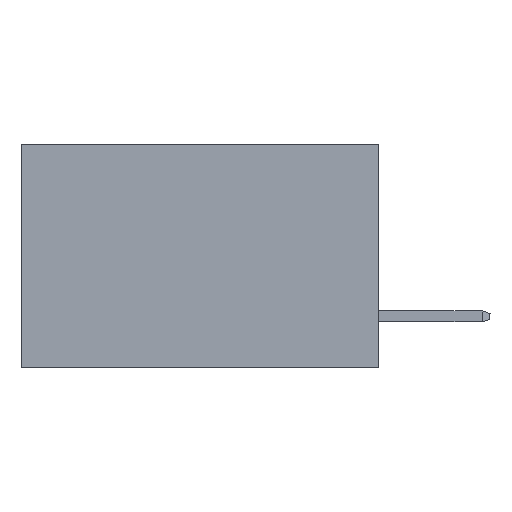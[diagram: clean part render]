
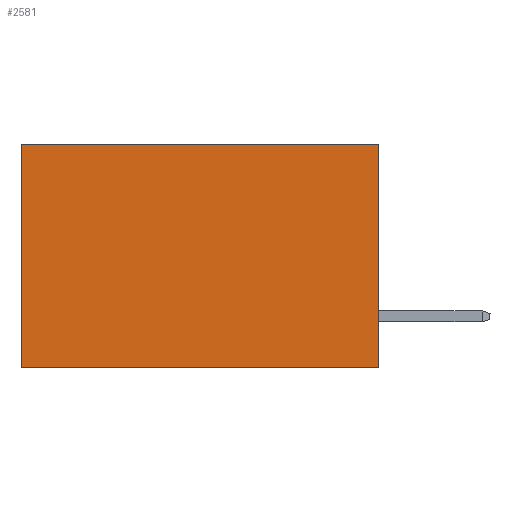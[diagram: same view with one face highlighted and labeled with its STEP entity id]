
A CAD part, left-side view. The second image highlights one B-rep face of the part: STEP entity #2581.
In plain terms, the highlighted planar face has unit normal (-1, 0, 0).
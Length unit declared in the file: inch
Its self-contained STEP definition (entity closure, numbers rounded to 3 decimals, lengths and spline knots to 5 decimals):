
#234 = VECTOR ( 'NONE', #2726, 39.37008 ) ;
#362 = LINE ( 'NONE', #3581, #11750 ) ;
#1575 = CARTESIAN_POINT ( 'NONE',  ( 0.277, 0.59, -0.37 ) ) ;
#2105 = CARTESIAN_POINT ( 'NONE',  ( 0.277, 0., -0.37 ) ) ;
#2530 = LINE ( 'NONE', #1575, #12619 ) ;
#2581 = ADVANCED_FACE ( 'NONE', ( #6671 ), #10044, .F. ) ;
#2726 = DIRECTION ( 'NONE',  ( 0., 1., 0. ) ) ;
#2768 = CARTESIAN_POINT ( 'NONE',  ( 0.277, 0., -0.37 ) ) ;
#3108 = DIRECTION ( 'NONE',  ( 1., 0., 0. ) ) ;
#3581 = CARTESIAN_POINT ( 'NONE',  ( 0.277, 0., 0. ) ) ;
#3671 = ORIENTED_EDGE ( 'NONE', *, *, #13797, .T. ) ;
#4850 = VERTEX_POINT ( 'NONE', #13586 ) ;
#5999 = DIRECTION ( 'NONE',  ( 0., 0., -1. ) ) ;
#6671 = FACE_OUTER_BOUND ( 'NONE', #15128, .T. ) ;
#9146 = ORIENTED_EDGE ( 'NONE', *, *, #15435, .T. ) ;
#9455 = VECTOR ( 'NONE', #5999, 39.37008 ) ;
#9879 = EDGE_CURVE ( 'NONE', #17568, #17441, #11213, .T. ) ;
#10044 = PLANE ( 'NONE',  #16343 ) ;
#11213 = LINE ( 'NONE', #2768, #234 ) ;
#11366 = CARTESIAN_POINT ( 'NONE',  ( 0.277, 0., 0. ) ) ;
#11750 = VECTOR ( 'NONE', #13020, 39.37008 ) ;
#12528 = DIRECTION ( 'NONE',  ( 0., 0., -1. ) ) ;
#12619 = VECTOR ( 'NONE', #12528, 39.37008 ) ;
#13012 = LINE ( 'NONE', #15502, #9455 ) ;
#13020 = DIRECTION ( 'NONE',  ( 0., 1., 0. ) ) ;
#13586 = CARTESIAN_POINT ( 'NONE',  ( 0.277, 0.59, 0. ) ) ;
#13797 = EDGE_CURVE ( 'NONE', #4850, #17441, #2530, .T. ) ;
#13886 = VERTEX_POINT ( 'NONE', #11366 ) ;
#14573 = CARTESIAN_POINT ( 'NONE',  ( 0.277, 0., -0.37 ) ) ;
#15128 = EDGE_LOOP ( 'NONE', ( #3671, #15467, #15903, #9146 ) ) ;
#15301 = EDGE_CURVE ( 'NONE', #13886, #17568, #13012, .T. ) ;
#15435 = EDGE_CURVE ( 'NONE', #13886, #4850, #362, .T. ) ;
#15467 = ORIENTED_EDGE ( 'NONE', *, *, #9879, .F. ) ;
#15502 = CARTESIAN_POINT ( 'NONE',  ( 0.277, 0., -0.37 ) ) ;
#15621 = CARTESIAN_POINT ( 'NONE',  ( 0.277, 0.59, -0.37 ) ) ;
#15903 = ORIENTED_EDGE ( 'NONE', *, *, #15301, .F. ) ;
#16343 = AXIS2_PLACEMENT_3D ( 'NONE', #2105, #3108, #16955 ) ;
#16955 = DIRECTION ( 'NONE',  ( 0., 0., -1. ) ) ;
#17441 = VERTEX_POINT ( 'NONE', #15621 ) ;
#17568 = VERTEX_POINT ( 'NONE', #14573 ) ;
